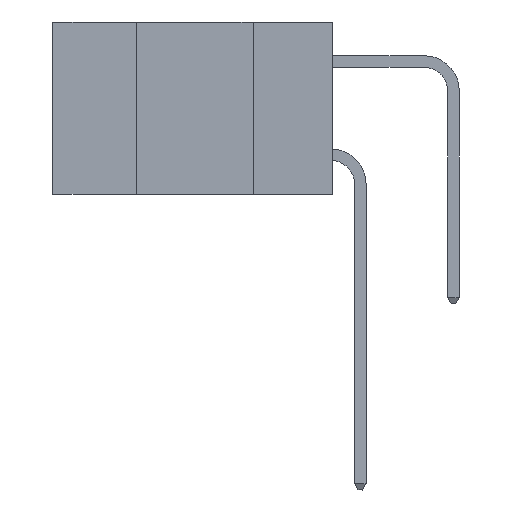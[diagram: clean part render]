
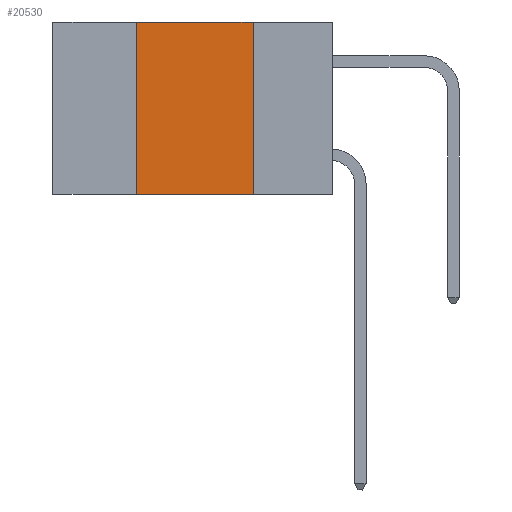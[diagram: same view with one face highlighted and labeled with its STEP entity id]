
A CAD part, left-side view. The second image highlights one B-rep face of the part: STEP entity #20530.
In plain terms, the highlighted planar face has unit normal (-1, 0, 0).
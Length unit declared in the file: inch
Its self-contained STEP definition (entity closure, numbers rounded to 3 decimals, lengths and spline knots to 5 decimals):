
#689 = EDGE_CURVE ( 'NONE', #14066, #14172, #5610, .T. ) ;
#1143 = CARTESIAN_POINT ( 'NONE',  ( 0., 0.42, 0. ) ) ;
#2216 = CARTESIAN_POINT ( 'NONE',  ( 0., 0.42, -0.37 ) ) ;
#2977 = VECTOR ( 'NONE', #13968, 39.37008 ) ;
#3125 = VECTOR ( 'NONE', #14928, 39.37008 ) ;
#3764 = CARTESIAN_POINT ( 'NONE',  ( 0., 0.6, 0. ) ) ;
#3836 = DIRECTION ( 'NONE',  ( 0., 0., -1. ) ) ;
#4192 = EDGE_CURVE ( 'NONE', #14172, #18276, #6777, .T. ) ;
#5052 = EDGE_CURVE ( 'NONE', #17167, #14066, #7385, .T. ) ;
#5610 = LINE ( 'NONE', #15955, #18392 ) ;
#5712 = EDGE_LOOP ( 'NONE', ( #15166, #9053, #20689, #14327 ) ) ;
#6014 = FACE_OUTER_BOUND ( 'NONE', #5712, .T. ) ;
#6226 = DIRECTION ( 'NONE',  ( 0., -1., 0. ) ) ;
#6711 = DIRECTION ( 'NONE',  ( 0., -1., 0. ) ) ;
#6777 = LINE ( 'NONE', #11353, #3125 ) ;
#7385 = LINE ( 'NONE', #1143, #2977 ) ;
#8957 = EDGE_CURVE ( 'NONE', #17167, #18276, #12643, .T. ) ;
#9053 = ORIENTED_EDGE ( 'NONE', *, *, #689, .F. ) ;
#10690 = AXIS2_PLACEMENT_3D ( 'NONE', #3764, #13761, #3836 ) ;
#11353 = CARTESIAN_POINT ( 'NONE',  ( 0., 0.17, 0. ) ) ;
#12643 = LINE ( 'NONE', #14816, #16326 ) ;
#13761 = DIRECTION ( 'NONE',  ( 1., 0., 0. ) ) ;
#13765 = CARTESIAN_POINT ( 'NONE',  ( 0., 0.17, 0. ) ) ;
#13968 = DIRECTION ( 'NONE',  ( 0., 0., 1. ) ) ;
#14066 = VERTEX_POINT ( 'NONE', #15233 ) ;
#14172 = VERTEX_POINT ( 'NONE', #13765 ) ;
#14327 = ORIENTED_EDGE ( 'NONE', *, *, #8957, .T. ) ;
#14816 = CARTESIAN_POINT ( 'NONE',  ( 0., 0.6, -0.37 ) ) ;
#14824 = CARTESIAN_POINT ( 'NONE',  ( 0., 0.17, -0.37 ) ) ;
#14928 = DIRECTION ( 'NONE',  ( 0., 0., -1. ) ) ;
#15166 = ORIENTED_EDGE ( 'NONE', *, *, #4192, .F. ) ;
#15233 = CARTESIAN_POINT ( 'NONE',  ( 0., 0.42, 0. ) ) ;
#15955 = CARTESIAN_POINT ( 'NONE',  ( 0., 0.6, 0. ) ) ;
#16326 = VECTOR ( 'NONE', #6711, 39.37008 ) ;
#17167 = VERTEX_POINT ( 'NONE', #2216 ) ;
#18276 = VERTEX_POINT ( 'NONE', #14824 ) ;
#18392 = VECTOR ( 'NONE', #6226, 39.37008 ) ;
#20399 = PLANE ( 'NONE',  #10690 ) ;
#20530 = ADVANCED_FACE ( 'NONE', ( #6014 ), #20399, .F. ) ;
#20689 = ORIENTED_EDGE ( 'NONE', *, *, #5052, .F. ) ;
